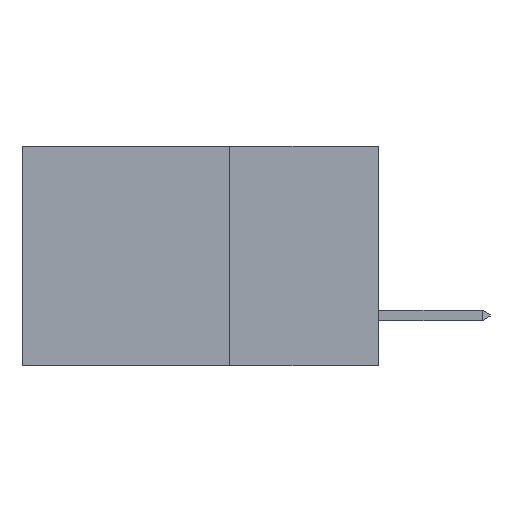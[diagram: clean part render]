
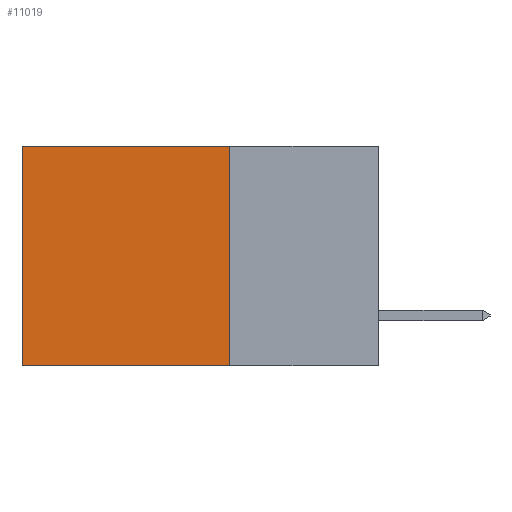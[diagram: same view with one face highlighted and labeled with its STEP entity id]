
A CAD part, left-side view. The second image highlights one B-rep face of the part: STEP entity #11019.
In plain terms, the highlighted planar face has unit normal (-1, 0, 0).
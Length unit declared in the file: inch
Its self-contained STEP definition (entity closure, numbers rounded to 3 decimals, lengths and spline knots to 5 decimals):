
#322 = CARTESIAN_POINT ( 'NONE',  ( 0.2615, 0.6, 0. ) ) ;
#400 = DIRECTION ( 'NONE',  ( 0., 0., -1. ) ) ;
#1256 = CARTESIAN_POINT ( 'NONE',  ( 0.2615, 0.25, -0.37 ) ) ;
#1338 = VECTOR ( 'NONE', #400, 39.37008 ) ;
#1577 = DIRECTION ( 'NONE',  ( 0., 0., -1. ) ) ;
#3527 = ORIENTED_EDGE ( 'NONE', *, *, #14995, .T. ) ;
#4210 = AXIS2_PLACEMENT_3D ( 'NONE', #20837, #12169, #8260 ) ;
#5134 = LINE ( 'NONE', #5946, #1338 ) ;
#5519 = LINE ( 'NONE', #1256, #17749 ) ;
#5573 = LINE ( 'NONE', #23892, #15124 ) ;
#5946 = CARTESIAN_POINT ( 'NONE',  ( 0.2615, 0.6, -0.37 ) ) ;
#6760 = VERTEX_POINT ( 'NONE', #20467 ) ;
#7329 = DIRECTION ( 'NONE',  ( 0., 1., 0. ) ) ;
#7557 = CARTESIAN_POINT ( 'NONE',  ( 0.2615, 0.25, 0. ) ) ;
#8260 = DIRECTION ( 'NONE',  ( 0., 0., -1. ) ) ;
#9073 = ORIENTED_EDGE ( 'NONE', *, *, #19435, .F. ) ;
#9128 = PLANE ( 'NONE',  #4210 ) ;
#9153 = VERTEX_POINT ( 'NONE', #12573 ) ;
#9636 = EDGE_CURVE ( 'NONE', #6760, #21748, #23437, .T. ) ;
#10656 = FACE_OUTER_BOUND ( 'NONE', #15215, .T. ) ;
#11019 = ADVANCED_FACE ( 'NONE', ( #10656 ), #9128, .F. ) ;
#12169 = DIRECTION ( 'NONE',  ( 1., 0., 0. ) ) ;
#12573 = CARTESIAN_POINT ( 'NONE',  ( 0.2615, 0.25, -0.37 ) ) ;
#13157 = VECTOR ( 'NONE', #7329, 39.37008 ) ;
#14523 = DIRECTION ( 'NONE',  ( 0., 1., 0. ) ) ;
#14995 = EDGE_CURVE ( 'NONE', #21748, #20350, #5134, .T. ) ;
#15124 = VECTOR ( 'NONE', #1577, 39.37008 ) ;
#15215 = EDGE_LOOP ( 'NONE', ( #3527, #9073, #18040, #21821 ) ) ;
#17749 = VECTOR ( 'NONE', #14523, 39.37008 ) ;
#18040 = ORIENTED_EDGE ( 'NONE', *, *, #19553, .F. ) ;
#19435 = EDGE_CURVE ( 'NONE', #9153, #20350, #5519, .T. ) ;
#19553 = EDGE_CURVE ( 'NONE', #6760, #9153, #5573, .T. ) ;
#20350 = VERTEX_POINT ( 'NONE', #20743 ) ;
#20467 = CARTESIAN_POINT ( 'NONE',  ( 0.2615, 0.25, 0. ) ) ;
#20743 = CARTESIAN_POINT ( 'NONE',  ( 0.2615, 0.6, -0.37 ) ) ;
#20837 = CARTESIAN_POINT ( 'NONE',  ( 0.2615, 0.25, -0.37 ) ) ;
#21748 = VERTEX_POINT ( 'NONE', #322 ) ;
#21821 = ORIENTED_EDGE ( 'NONE', *, *, #9636, .T. ) ;
#23437 = LINE ( 'NONE', #7557, #13157 ) ;
#23892 = CARTESIAN_POINT ( 'NONE',  ( 0.2615, 0.25, -0.37 ) ) ;
